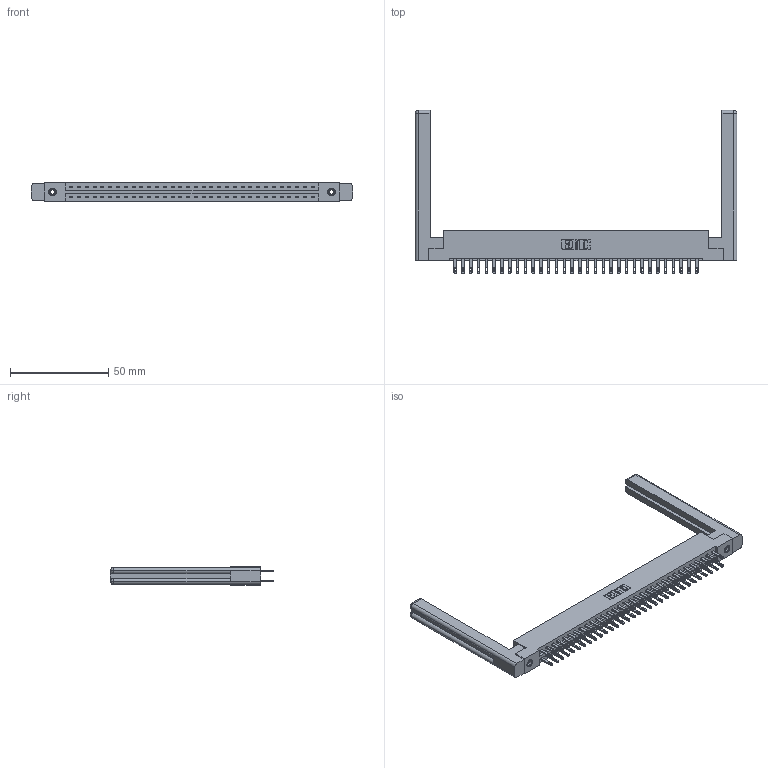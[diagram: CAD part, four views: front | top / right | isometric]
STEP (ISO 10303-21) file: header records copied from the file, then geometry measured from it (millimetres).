
FILE_DESCRIPTION (( 'STEP AP203' ), '1' );
FILE_NAME ('337-064-500-258.STEP', '2019-10-09T21:53:21', ( '' ), ( '' ), 'SwSTEP 2.0', 'SolidWorks 2016', '' );
FILE_SCHEMA (( 'CONFIG_CONTROL_DESIGN' ));
Length unit declared in the file: inch
Products named in the file (5): 337 Part_Flush Mounting Lugs - 0.156 Dia-TI; 345-292-001_345-293-100; 345-250-001_345-250-001-102; 337-064-500-258; 307-220-058
Assembly tree (69 placements, depth 2):
  337-064-500-258
    337 Part_Flush Mounting Lugs - 0.156 Dia-TI
    345-292-001_345-293-100  x64
    345-250-001_345-250-001-102  x2
    307-220-058  x2
Bounding box: 163.42 x 82.94 x 9.4 mm (x, y, z)
Volume: 24427.7 mm3; surface area: 25200.9 mm2
Topology: 69 solids, 69 shells, 3456 faces, 10457 edges, 6958 vertices
Faces by surface type: plane 2202, cylinder 1230, cone 12, torus 12
Entity records: 28668 total; most frequent: CARTESIAN_POINT 4845, ORIENTED_EDGE 4720, DIRECTION 4156, EDGE_CURVE 2360, VECTOR 2180, LINE 2180, VERTEX_POINT 1566, AXIS2_PLACEMENT_3D 988
